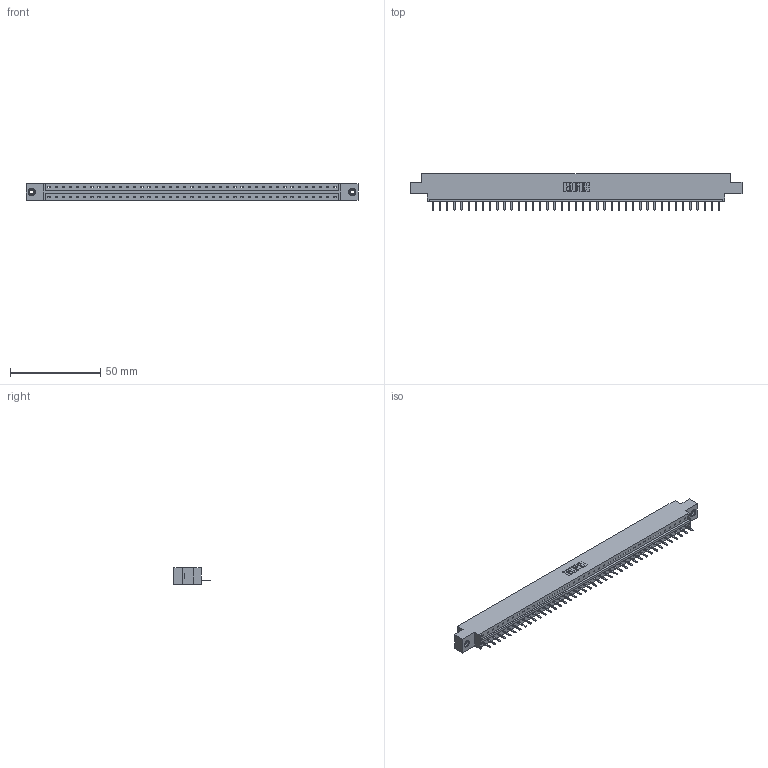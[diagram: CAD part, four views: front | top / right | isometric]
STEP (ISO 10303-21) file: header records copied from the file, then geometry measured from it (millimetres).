
FILE_DESCRIPTION (( 'STEP AP203' ), '1' );
FILE_NAME ('833-041-520-608.STEP', '2020-06-03T18:42:04', ( '' ), ( '' ), 'SwSTEP 2.0', 'SolidWorks 2020', '' );
FILE_SCHEMA (( 'CONFIG_CONTROL_DESIGN' ));
Length unit declared in the file: inch
Products named in the file (4): 833-041-520-608; 345-250-001_345-250-003-102; 833 Part_Offset - .156 Dia - TI; 345-292-001_345-293-120
Assembly tree (44 placements, depth 2):
  833-041-520-608
    833 Part_Offset - .156 Dia - TI
    345-292-001_345-293-120  x41
    345-250-001_345-250-003-102  x2
Bounding box: 184 x 20.02 x 9.4 mm (x, y, z)
Volume: 18154.5 mm3; surface area: 19446.5 mm2
Topology: 44 solids, 44 shells, 2720 faces, 8003 edges, 5218 vertices
Faces by surface type: plane 1910, cylinder 794, cone 12, torus 4
Entity records: 26626 total; most frequent: CARTESIAN_POINT 4588, ORIENTED_EDGE 4546, DIRECTION 3893, EDGE_CURVE 2273, LINE 2121, VECTOR 2121, VERTEX_POINT 1508, AXIS2_PLACEMENT_3D 886
